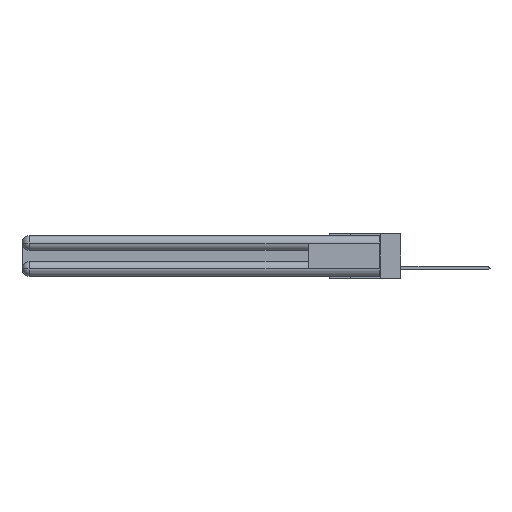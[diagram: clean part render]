
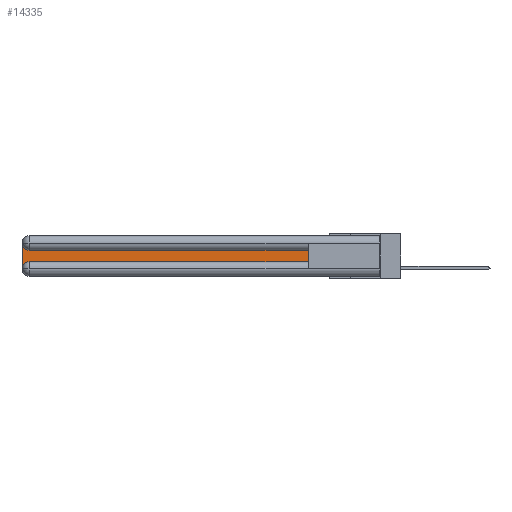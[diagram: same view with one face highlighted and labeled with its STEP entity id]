
A CAD part, left-side view. The second image highlights one B-rep face of the part: STEP entity #14335.
In plain terms, the highlighted planar face has unit normal (-1, 0, 0).
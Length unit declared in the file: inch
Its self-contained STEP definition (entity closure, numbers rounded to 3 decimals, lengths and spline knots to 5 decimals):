
#434 = AXIS2_PLACEMENT_3D ( 'NONE', #28761, #8055, #29101 ) ;
#909 = ORIENTED_EDGE ( 'NONE', *, *, #8517, .T. ) ;
#1254 = DIRECTION ( 'NONE',  ( 0., 0., -1. ) ) ;
#1586 = VERTEX_POINT ( 'NONE', #3527 ) ;
#2612 = LINE ( 'NONE', #31503, #29545 ) ;
#3524 = ORIENTED_EDGE ( 'NONE', *, *, #13239, .T. ) ;
#3527 = CARTESIAN_POINT ( 'NONE',  ( 0.075, 3., -0.0625 ) ) ;
#3670 = LINE ( 'NONE', #27488, #30623 ) ;
#5358 = CARTESIAN_POINT ( 'NONE',  ( 0.075, 2.94, -0.2175 ) ) ;
#5803 = LINE ( 'NONE', #19156, #7469 ) ;
#7303 = EDGE_CURVE ( 'NONE', #10453, #1586, #23783, .T. ) ;
#7469 = VECTOR ( 'NONE', #16538, 39.37008 ) ;
#7797 = FACE_OUTER_BOUND ( 'NONE', #10648, .T. ) ;
#8055 = DIRECTION ( 'NONE',  ( 1., 0., 0. ) ) ;
#8383 = VERTEX_POINT ( 'NONE', #5358 ) ;
#8517 = EDGE_CURVE ( 'NONE', #16081, #14145, #3670, .T. ) ;
#8540 = CARTESIAN_POINT ( 'NONE',  ( 0.075, 3., -0.2775 ) ) ;
#8844 = PLANE ( 'NONE',  #21262 ) ;
#9210 = CARTESIAN_POINT ( 'NONE',  ( 0.075, 0.6, -0.1225 ) ) ;
#9411 = DIRECTION ( 'NONE',  ( 1., 0., 0. ) ) ;
#9730 = ORIENTED_EDGE ( 'NONE', *, *, #10953, .T. ) ;
#10453 = VERTEX_POINT ( 'NONE', #31709 ) ;
#10647 = CARTESIAN_POINT ( 'NONE',  ( 0.075, 3., -0.2175 ) ) ;
#10648 = EDGE_LOOP ( 'NONE', ( #28348, #19945, #11481, #9730, #3524, #909 ) ) ;
#10953 = EDGE_CURVE ( 'NONE', #12373, #8383, #12540, .T. ) ;
#11481 = ORIENTED_EDGE ( 'NONE', *, *, #32206, .T. ) ;
#11868 = DIRECTION ( 'NONE',  ( 0., 0., 1. ) ) ;
#12373 = VERTEX_POINT ( 'NONE', #8540 ) ;
#12540 = CIRCLE ( 'NONE', #434, 0.06 ) ;
#13239 = EDGE_CURVE ( 'NONE', #8383, #16081, #5803, .T. ) ;
#14145 = VERTEX_POINT ( 'NONE', #9210 ) ;
#14335 = ADVANCED_FACE ( 'NONE', ( #7797 ), #8844, .F. ) ;
#14863 = DIRECTION ( 'NONE',  ( 0., 0., -1. ) ) ;
#16081 = VERTEX_POINT ( 'NONE', #27527 ) ;
#16538 = DIRECTION ( 'NONE',  ( 0., -1., 0. ) ) ;
#16951 = VECTOR ( 'NONE', #23393, 39.37008 ) ;
#17369 = CARTESIAN_POINT ( 'NONE',  ( 0.075, 2.94, -0.0625 ) ) ;
#17861 = AXIS2_PLACEMENT_3D ( 'NONE', #17369, #9411, #14863 ) ;
#18284 = DIRECTION ( 'NONE',  ( 0., 1., 0. ) ) ;
#19156 = CARTESIAN_POINT ( 'NONE',  ( 0.075, 0.6, -0.2175 ) ) ;
#19805 = LINE ( 'NONE', #10647, #16951 ) ;
#19945 = ORIENTED_EDGE ( 'NONE', *, *, #7303, .T. ) ;
#21262 = AXIS2_PLACEMENT_3D ( 'NONE', #24349, #21618, #1254 ) ;
#21618 = DIRECTION ( 'NONE',  ( 1., 0., 0. ) ) ;
#23393 = DIRECTION ( 'NONE',  ( 0., 0., -1. ) ) ;
#23783 = CIRCLE ( 'NONE', #17861, 0.06 ) ;
#24349 = CARTESIAN_POINT ( 'NONE',  ( 0.075, 3., -0.1225 ) ) ;
#25443 = EDGE_CURVE ( 'NONE', #14145, #10453, #2612, .T. ) ;
#27488 = CARTESIAN_POINT ( 'NONE',  ( 0.075, 0.6, -0.2175 ) ) ;
#27527 = CARTESIAN_POINT ( 'NONE',  ( 0.075, 0.6, -0.2175 ) ) ;
#28348 = ORIENTED_EDGE ( 'NONE', *, *, #25443, .T. ) ;
#28761 = CARTESIAN_POINT ( 'NONE',  ( 0.075, 2.94, -0.2775 ) ) ;
#29101 = DIRECTION ( 'NONE',  ( 0., 0., -1. ) ) ;
#29545 = VECTOR ( 'NONE', #18284, 39.37008 ) ;
#30623 = VECTOR ( 'NONE', #11868, 39.37008 ) ;
#31503 = CARTESIAN_POINT ( 'NONE',  ( 0.075, 0.6, -0.1225 ) ) ;
#31709 = CARTESIAN_POINT ( 'NONE',  ( 0.075, 2.94, -0.1225 ) ) ;
#32206 = EDGE_CURVE ( 'NONE', #1586, #12373, #19805, .T. ) ;
